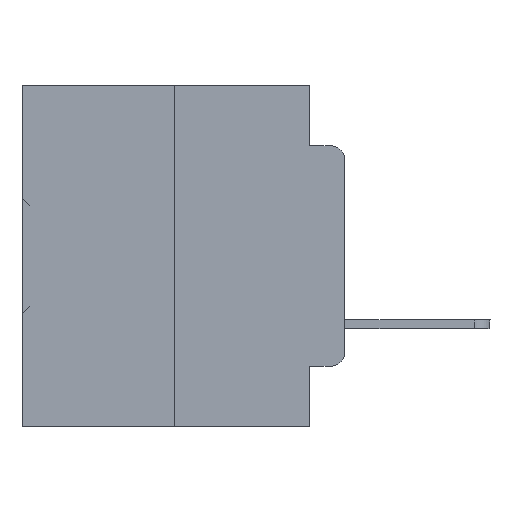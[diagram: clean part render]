
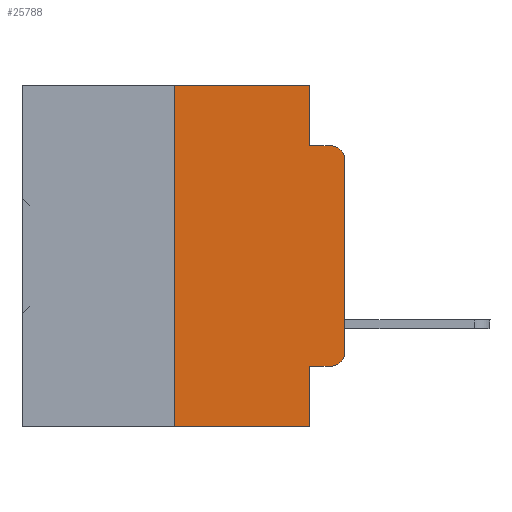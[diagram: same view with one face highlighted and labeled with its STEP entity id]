
A CAD part, left-side view. The second image highlights one B-rep face of the part: STEP entity #25788.
In plain terms, the highlighted planar face has unit normal (-1, 0, 0).
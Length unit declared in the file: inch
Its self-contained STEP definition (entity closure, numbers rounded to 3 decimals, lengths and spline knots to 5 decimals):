
#301 = EDGE_CURVE ( 'NONE', #18440, #37705, #21529, .T. ) ;
#1524 = ORIENTED_EDGE ( 'NONE', *, *, #14806, .F. ) ;
#1545 = CARTESIAN_POINT ( 'NONE',  ( 0., 0., 0. ) ) ;
#2187 = EDGE_CURVE ( 'NONE', #29608, #27233, #35380, .T. ) ;
#2774 = AXIS2_PLACEMENT_3D ( 'NONE', #11261, #22414, #7547 ) ;
#2836 = EDGE_LOOP ( 'NONE', ( #13853, #10878, #34142, #28710, #1524, #35142, #4262, #9810, #18369, #36263 ) ) ;
#2871 = CARTESIAN_POINT ( 'NONE',  ( 0., 0.051, -0.5 ) ) ;
#3043 = LINE ( 'NONE', #27052, #7977 ) ;
#3838 = CARTESIAN_POINT ( 'NONE',  ( 0., 0.051, -0.0885 ) ) ;
#4262 = ORIENTED_EDGE ( 'NONE', *, *, #301, .T. ) ;
#4921 = EDGE_CURVE ( 'NONE', #18440, #27540, #3043, .T. ) ;
#5014 = FACE_OUTER_BOUND ( 'NONE', #2836, .T. ) ;
#5060 = LINE ( 'NONE', #1545, #26125 ) ;
#5350 = EDGE_CURVE ( 'NONE', #15161, #32649, #35639, .T. ) ;
#6085 = VECTOR ( 'NONE', #11858, 39.37008 ) ;
#7150 = EDGE_CURVE ( 'NONE', #27233, #7886, #5060, .T. ) ;
#7205 = DIRECTION ( 'NONE',  ( 0., 0., -1. ) ) ;
#7423 = CARTESIAN_POINT ( 'NONE',  ( 0., 0.02, -0.4115 ) ) ;
#7547 = DIRECTION ( 'NONE',  ( 0., 0., -1. ) ) ;
#7886 = VERTEX_POINT ( 'NONE', #22119 ) ;
#7977 = VECTOR ( 'NONE', #12008, 39.37008 ) ;
#8033 = DIRECTION ( 'NONE',  ( -1., 0., 0. ) ) ;
#8069 = CARTESIAN_POINT ( 'NONE',  ( 0., 0.02, -0.0885 ) ) ;
#8270 = CARTESIAN_POINT ( 'NONE',  ( 0., 0.051, -0.4115 ) ) ;
#8637 = VECTOR ( 'NONE', #14912, 39.37008 ) ;
#9743 = CARTESIAN_POINT ( 'NONE',  ( 0., 0.473, 0. ) ) ;
#9810 = ORIENTED_EDGE ( 'NONE', *, *, #31713, .F. ) ;
#10127 = VERTEX_POINT ( 'NONE', #8270 ) ;
#10878 = ORIENTED_EDGE ( 'NONE', *, *, #13454, .T. ) ;
#11261 = CARTESIAN_POINT ( 'NONE',  ( 0., 0.473, 0. ) ) ;
#11305 = DIRECTION ( 'NONE',  ( 0., 0., 1. ) ) ;
#11858 = DIRECTION ( 'NONE',  ( 0., 0., -1. ) ) ;
#11900 = LINE ( 'NONE', #12468, #28420 ) ;
#12008 = DIRECTION ( 'NONE',  ( 0., 0., 1. ) ) ;
#12346 = CARTESIAN_POINT ( 'NONE',  ( 0., 0.051, -0.0885 ) ) ;
#12360 = DIRECTION ( 'NONE',  ( 0., -1., 0. ) ) ;
#12468 = CARTESIAN_POINT ( 'NONE',  ( 0., 0.051, 0. ) ) ;
#13454 = EDGE_CURVE ( 'NONE', #7886, #32649, #24735, .T. ) ;
#13853 = ORIENTED_EDGE ( 'NONE', *, *, #7150, .T. ) ;
#14806 = EDGE_CURVE ( 'NONE', #27540, #18515, #33614, .T. ) ;
#14912 = DIRECTION ( 'NONE',  ( 0., -1., 0. ) ) ;
#15032 = DIRECTION ( 'NONE',  ( 0., 0., -1. ) ) ;
#15161 = VERTEX_POINT ( 'NONE', #3838 ) ;
#15288 = CARTESIAN_POINT ( 'NONE',  ( 0., 0.473, -0.5 ) ) ;
#18369 = ORIENTED_EDGE ( 'NONE', *, *, #33588, .T. ) ;
#18440 = VERTEX_POINT ( 'NONE', #26006 ) ;
#18515 = VERTEX_POINT ( 'NONE', #23467 ) ;
#19537 = CARTESIAN_POINT ( 'NONE',  ( 0., 0.02, -0.3915 ) ) ;
#19949 = CARTESIAN_POINT ( 'NONE',  ( 0., 0.02, -0.1085 ) ) ;
#20417 = CARTESIAN_POINT ( 'NONE',  ( 0., 0.25, 0. ) ) ;
#20669 = DIRECTION ( 'NONE',  ( 0., -1., 0. ) ) ;
#21529 = LINE ( 'NONE', #15288, #22023 ) ;
#21677 = DIRECTION ( 'NONE',  ( 0., -1., 0. ) ) ;
#22023 = VECTOR ( 'NONE', #12360, 39.37008 ) ;
#22119 = CARTESIAN_POINT ( 'NONE',  ( 0., 0., -0.1085 ) ) ;
#22414 = DIRECTION ( 'NONE',  ( 1., 0., 0. ) ) ;
#23467 = CARTESIAN_POINT ( 'NONE',  ( 0., 0.051, 0. ) ) ;
#24735 = CIRCLE ( 'NONE', #27955, 0.02 ) ;
#24915 = CARTESIAN_POINT ( 'NONE',  ( 0., 0., -0.3915 ) ) ;
#25788 = ADVANCED_FACE ( 'NONE', ( #5014 ), #38042, .F. ) ;
#26006 = CARTESIAN_POINT ( 'NONE',  ( 0., 0.25, -0.5 ) ) ;
#26125 = VECTOR ( 'NONE', #11305, 39.37008 ) ;
#26734 = CARTESIAN_POINT ( 'NONE',  ( 0., 0.051, -0.4115 ) ) ;
#27052 = CARTESIAN_POINT ( 'NONE',  ( 0., 0.25, 0. ) ) ;
#27233 = VERTEX_POINT ( 'NONE', #24915 ) ;
#27540 = VERTEX_POINT ( 'NONE', #20417 ) ;
#27955 = AXIS2_PLACEMENT_3D ( 'NONE', #19949, #8033, #37728 ) ;
#28420 = VECTOR ( 'NONE', #15032, 39.37008 ) ;
#28710 = ORIENTED_EDGE ( 'NONE', *, *, #37236, .F. ) ;
#29120 = AXIS2_PLACEMENT_3D ( 'NONE', #19537, #31452, #7205 ) ;
#29274 = LINE ( 'NONE', #26734, #37412 ) ;
#29458 = LINE ( 'NONE', #38644, #6085 ) ;
#29608 = VERTEX_POINT ( 'NONE', #7423 ) ;
#31452 = DIRECTION ( 'NONE',  ( -1., 0., 0. ) ) ;
#31713 = EDGE_CURVE ( 'NONE', #10127, #37705, #29458, .T. ) ;
#32649 = VERTEX_POINT ( 'NONE', #8069 ) ;
#33588 = EDGE_CURVE ( 'NONE', #10127, #29608, #29274, .T. ) ;
#33614 = LINE ( 'NONE', #9743, #37809 ) ;
#34142 = ORIENTED_EDGE ( 'NONE', *, *, #5350, .F. ) ;
#35142 = ORIENTED_EDGE ( 'NONE', *, *, #4921, .F. ) ;
#35380 = CIRCLE ( 'NONE', #29120, 0.02 ) ;
#35639 = LINE ( 'NONE', #12346, #8637 ) ;
#36263 = ORIENTED_EDGE ( 'NONE', *, *, #2187, .T. ) ;
#37236 = EDGE_CURVE ( 'NONE', #18515, #15161, #11900, .T. ) ;
#37412 = VECTOR ( 'NONE', #20669, 39.37008 ) ;
#37705 = VERTEX_POINT ( 'NONE', #2871 ) ;
#37728 = DIRECTION ( 'NONE',  ( 0., 0., -1. ) ) ;
#37809 = VECTOR ( 'NONE', #21677, 39.37008 ) ;
#38042 = PLANE ( 'NONE',  #2774 ) ;
#38644 = CARTESIAN_POINT ( 'NONE',  ( 0., 0.051, 0. ) ) ;
